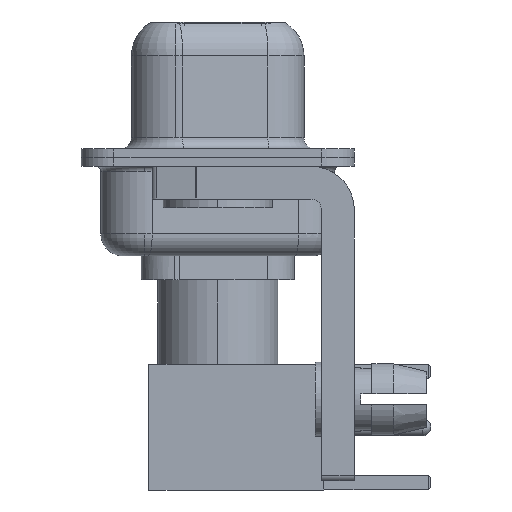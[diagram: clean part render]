
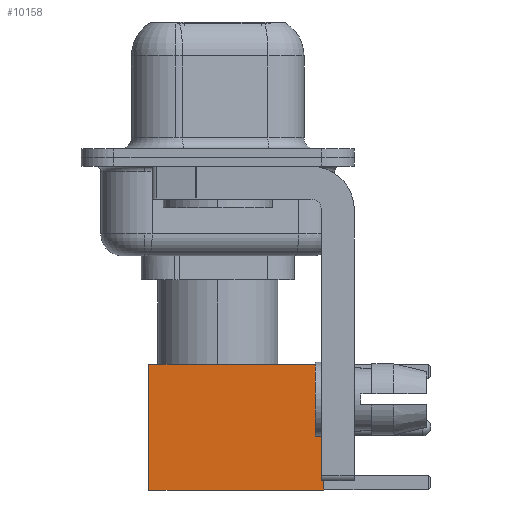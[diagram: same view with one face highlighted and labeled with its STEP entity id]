
A CAD part, left-side view. The second image highlights one B-rep face of the part: STEP entity #10158.
In plain terms, the highlighted face is planar.
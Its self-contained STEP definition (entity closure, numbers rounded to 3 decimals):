
#1211 = VERTEX_POINT ( 'NONE', #7102 ) ;
#1451 = CARTESIAN_POINT ( 'NONE',  ( -2.875, 2.875, 8. ) ) ;
#2093 = DIRECTION ( 'NONE',  ( -1., 0., 0. ) ) ;
#2275 = AXIS2_PLACEMENT_3D ( 'NONE', #8887, #18991, #4550 ) ;
#2598 = VERTEX_POINT ( 'NONE', #18156 ) ;
#2749 = VECTOR ( 'NONE', #13967, 1000. ) ;
#3502 = VERTEX_POINT ( 'NONE', #1451 ) ;
#3720 = LINE ( 'NONE', #10146, #15298 ) ;
#3961 = ORIENTED_EDGE ( 'NONE', *, *, #15527, .T. ) ;
#4550 = DIRECTION ( 'NONE',  ( 0., 0., 1. ) ) ;
#6470 = DIRECTION ( 'NONE',  ( 0., 0., -1. ) ) ;
#6489 = EDGE_LOOP ( 'NONE', ( #8450, #3961, #17962, #15428 ) ) ;
#7102 = CARTESIAN_POINT ( 'NONE',  ( 2.875, 2.875, 0. ) ) ;
#7659 = CARTESIAN_POINT ( 'NONE',  ( 0., 2.875, 0. ) ) ;
#8215 = LINE ( 'NONE', #11571, #14737 ) ;
#8450 = ORIENTED_EDGE ( 'NONE', *, *, #10825, .T. ) ;
#8887 = CARTESIAN_POINT ( 'NONE',  ( 2.875, 2.875, 0. ) ) ;
#9992 = LINE ( 'NONE', #11573, #12444 ) ;
#10146 = CARTESIAN_POINT ( 'NONE',  ( -2.875, 2.875, 0. ) ) ;
#10158 = ADVANCED_FACE ( 'NONE', ( #10663 ), #12561, .T. ) ;
#10663 = FACE_OUTER_BOUND ( 'NONE', #6489, .T. ) ;
#10825 = EDGE_CURVE ( 'NONE', #20273, #1211, #8215, .T. ) ;
#11571 = CARTESIAN_POINT ( 'NONE',  ( 2.875, 2.875, 0. ) ) ;
#11573 = CARTESIAN_POINT ( 'NONE',  ( 0., 2.875, 8. ) ) ;
#12223 = EDGE_CURVE ( 'NONE', #20273, #3502, #9992, .T. ) ;
#12444 = VECTOR ( 'NONE', #2093, 1000. ) ;
#12561 = PLANE ( 'NONE',  #2275 ) ;
#13967 = DIRECTION ( 'NONE',  ( -1., 0., 0. ) ) ;
#14737 = VECTOR ( 'NONE', #14938, 1000. ) ;
#14938 = DIRECTION ( 'NONE',  ( 0., 0., -1. ) ) ;
#15298 = VECTOR ( 'NONE', #6470, 1000. ) ;
#15428 = ORIENTED_EDGE ( 'NONE', *, *, #12223, .F. ) ;
#15527 = EDGE_CURVE ( 'NONE', #1211, #2598, #20806, .T. ) ;
#16155 = EDGE_CURVE ( 'NONE', #3502, #2598, #3720, .T. ) ;
#17659 = CARTESIAN_POINT ( 'NONE',  ( 2.875, 2.875, 8. ) ) ;
#17962 = ORIENTED_EDGE ( 'NONE', *, *, #16155, .F. ) ;
#18156 = CARTESIAN_POINT ( 'NONE',  ( -2.875, 2.875, 0. ) ) ;
#18991 = DIRECTION ( 'NONE',  ( 0., 1., 0. ) ) ;
#20273 = VERTEX_POINT ( 'NONE', #17659 ) ;
#20806 = LINE ( 'NONE', #7659, #2749 ) ;
